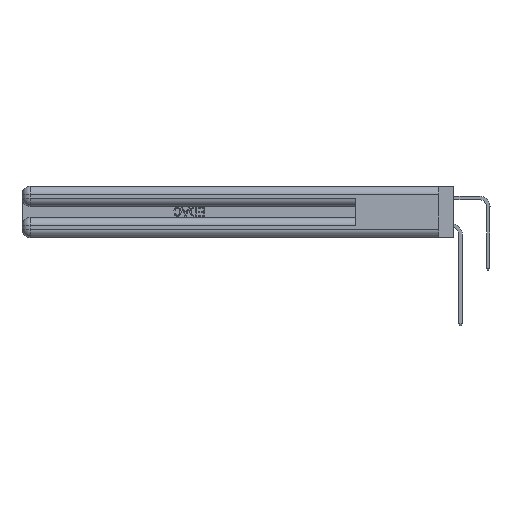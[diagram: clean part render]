
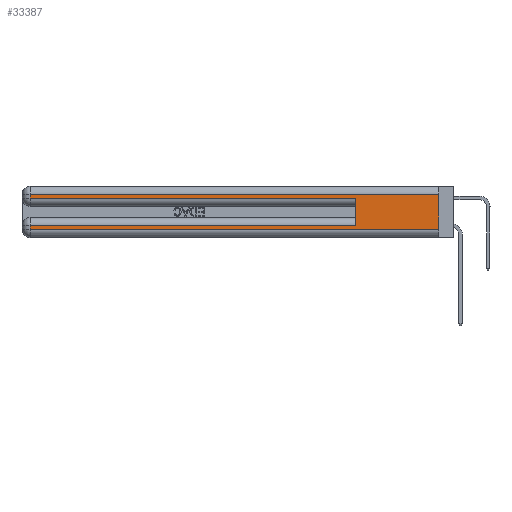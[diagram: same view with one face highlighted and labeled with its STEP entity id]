
A CAD part, left-side view. The second image highlights one B-rep face of the part: STEP entity #33387.
In plain terms, the highlighted planar face has unit normal (-1, 0, 0).
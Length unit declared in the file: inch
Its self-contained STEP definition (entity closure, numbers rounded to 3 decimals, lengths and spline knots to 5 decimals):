
#1085 = CARTESIAN_POINT ( 'NONE',  ( 0., 2.94, 0.31 ) ) ;
#1411 = DIRECTION ( 'NONE',  ( 0., 0., 1. ) ) ;
#1944 = CARTESIAN_POINT ( 'NONE',  ( 0., 0., 0.31 ) ) ;
#2486 = FACE_OUTER_BOUND ( 'NONE', #16882, .T. ) ;
#3302 = CARTESIAN_POINT ( 'NONE',  ( 0., 0., 0.285 ) ) ;
#3319 = ORIENTED_EDGE ( 'NONE', *, *, #27698, .T. ) ;
#4964 = EDGE_CURVE ( 'NONE', #41908, #20456, #17226, .T. ) ;
#5896 = CARTESIAN_POINT ( 'NONE',  ( 0., 0., 0.31 ) ) ;
#6396 = LINE ( 'NONE', #19840, #23676 ) ;
#6862 = EDGE_CURVE ( 'NONE', #8859, #31916, #27506, .T. ) ;
#7415 = VECTOR ( 'NONE', #20188, 39.37008 ) ;
#8859 = VERTEX_POINT ( 'NONE', #40078 ) ;
#9084 = CARTESIAN_POINT ( 'NONE',  ( 0., 2.94, 0.37 ) ) ;
#9466 = ORIENTED_EDGE ( 'NONE', *, *, #34016, .F. ) ;
#9818 = VECTOR ( 'NONE', #31511, 39.37008 ) ;
#9855 = EDGE_CURVE ( 'NONE', #11305, #44185, #27842, .T. ) ;
#10874 = ORIENTED_EDGE ( 'NONE', *, *, #11097, .F. ) ;
#11097 = EDGE_CURVE ( 'NONE', #8859, #17868, #6396, .T. ) ;
#11305 = VERTEX_POINT ( 'NONE', #28215 ) ;
#12009 = DIRECTION ( 'NONE',  ( 0., -1., 0. ) ) ;
#13425 = CARTESIAN_POINT ( 'NONE',  ( 0., 0., 0.06 ) ) ;
#13997 = VECTOR ( 'NONE', #18441, 39.37008 ) ;
#15903 = EDGE_CURVE ( 'NONE', #31916, #11305, #45667, .T. ) ;
#16315 = VECTOR ( 'NONE', #41229, 39.37008 ) ;
#16729 = DIRECTION ( 'NONE',  ( 1., 0., 0. ) ) ;
#16882 = EDGE_LOOP ( 'NONE', ( #9466, #40986, #29025, #3319, #10874, #22497, #40624, #26526 ) ) ;
#16963 = CARTESIAN_POINT ( 'NONE',  ( 0., 0., 0.085 ) ) ;
#17226 = LINE ( 'NONE', #9084, #7415 ) ;
#17701 = VECTOR ( 'NONE', #20672, 39.37008 ) ;
#17868 = VERTEX_POINT ( 'NONE', #22253 ) ;
#18441 = DIRECTION ( 'NONE',  ( 0., 0., -1. ) ) ;
#19840 = CARTESIAN_POINT ( 'NONE',  ( 0., 0.6, 0.145 ) ) ;
#20188 = DIRECTION ( 'NONE',  ( 0., 0., -1. ) ) ;
#20456 = VERTEX_POINT ( 'NONE', #29758 ) ;
#20672 = DIRECTION ( 'NONE',  ( 0., 1., 0. ) ) ;
#20709 = VERTEX_POINT ( 'NONE', #5896 ) ;
#21901 = LINE ( 'NONE', #3302, #30598 ) ;
#22253 = CARTESIAN_POINT ( 'NONE',  ( 0., 0.6, 0.285 ) ) ;
#22497 = ORIENTED_EDGE ( 'NONE', *, *, #6862, .T. ) ;
#23676 = VECTOR ( 'NONE', #1411, 39.37008 ) ;
#23793 = LINE ( 'NONE', #44148, #13997 ) ;
#25403 = DIRECTION ( 'NONE',  ( 0., -1., 0. ) ) ;
#26526 = ORIENTED_EDGE ( 'NONE', *, *, #9855, .T. ) ;
#27506 = LINE ( 'NONE', #16963, #17701 ) ;
#27527 = PLANE ( 'NONE',  #28058 ) ;
#27698 = EDGE_CURVE ( 'NONE', #20456, #17868, #21901, .T. ) ;
#27842 = LINE ( 'NONE', #41454, #46253 ) ;
#28058 = AXIS2_PLACEMENT_3D ( 'NONE', #38778, #16729, #42470 ) ;
#28215 = CARTESIAN_POINT ( 'NONE',  ( 0., 2.94, 0.06 ) ) ;
#29025 = ORIENTED_EDGE ( 'NONE', *, *, #4964, .T. ) ;
#29400 = LINE ( 'NONE', #1944, #9818 ) ;
#29758 = CARTESIAN_POINT ( 'NONE',  ( 0., 2.94, 0.285 ) ) ;
#30598 = VECTOR ( 'NONE', #25403, 39.37008 ) ;
#31511 = DIRECTION ( 'NONE',  ( 0., 1., 0. ) ) ;
#31916 = VERTEX_POINT ( 'NONE', #41142 ) ;
#33387 = ADVANCED_FACE ( 'NONE', ( #2486 ), #27527, .F. ) ;
#33847 = CARTESIAN_POINT ( 'NONE',  ( 0., 2.94, 0.37 ) ) ;
#34016 = EDGE_CURVE ( 'NONE', #20709, #44185, #23793, .T. ) ;
#35711 = EDGE_CURVE ( 'NONE', #20709, #41908, #29400, .T. ) ;
#38778 = CARTESIAN_POINT ( 'NONE',  ( 0., 0., 0.37 ) ) ;
#40078 = CARTESIAN_POINT ( 'NONE',  ( 0., 0.6, 0.085 ) ) ;
#40624 = ORIENTED_EDGE ( 'NONE', *, *, #15903, .T. ) ;
#40986 = ORIENTED_EDGE ( 'NONE', *, *, #35711, .T. ) ;
#41142 = CARTESIAN_POINT ( 'NONE',  ( 0., 2.94, 0.085 ) ) ;
#41229 = DIRECTION ( 'NONE',  ( 0., 0., -1. ) ) ;
#41454 = CARTESIAN_POINT ( 'NONE',  ( 0., 0., 0.06 ) ) ;
#41908 = VERTEX_POINT ( 'NONE', #1085 ) ;
#42470 = DIRECTION ( 'NONE',  ( 0., 0., -1. ) ) ;
#44148 = CARTESIAN_POINT ( 'NONE',  ( 0., 0., 0.37 ) ) ;
#44185 = VERTEX_POINT ( 'NONE', #13425 ) ;
#45667 = LINE ( 'NONE', #33847, #16315 ) ;
#46253 = VECTOR ( 'NONE', #12009, 39.37008 ) ;
